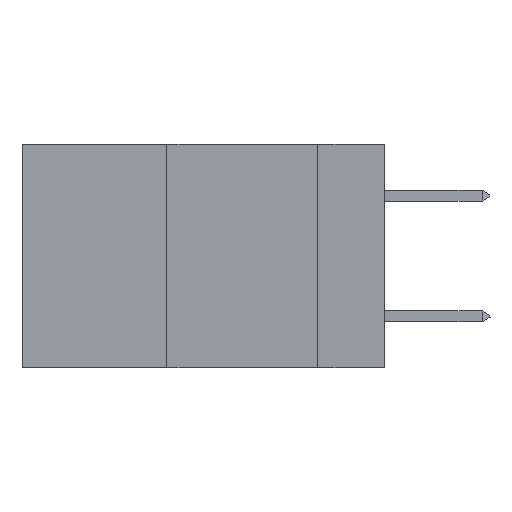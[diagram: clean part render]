
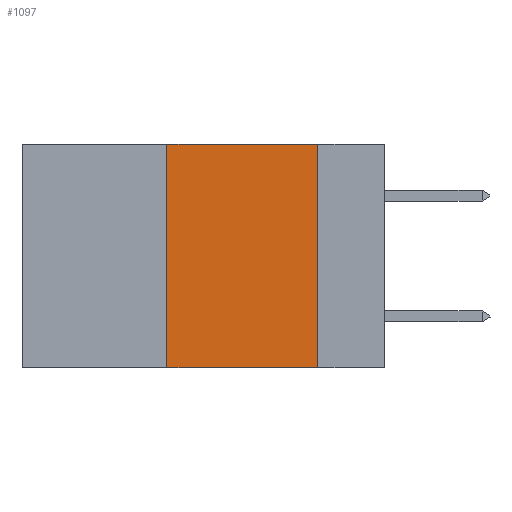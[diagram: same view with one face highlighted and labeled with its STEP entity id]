
A CAD part, left-side view. The second image highlights one B-rep face of the part: STEP entity #1097.
In plain terms, the highlighted planar face has unit normal (-1, 0, 0).
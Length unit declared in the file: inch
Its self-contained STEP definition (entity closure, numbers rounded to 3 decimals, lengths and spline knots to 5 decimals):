
#472 = CARTESIAN_POINT ( 'NONE',  ( 0., 0.36, 0. ) ) ;
#550 = VECTOR ( 'NONE', #9578, 39.37008 ) ;
#721 = VECTOR ( 'NONE', #6037, 39.37008 ) ;
#830 = EDGE_LOOP ( 'NONE', ( #2233, #8775, #4856, #7892 ) ) ;
#1097 = ADVANCED_FACE ( 'NONE', ( #7365 ), #3379, .F. ) ;
#1171 = EDGE_CURVE ( 'NONE', #7683, #2452, #3147, .T. ) ;
#1399 = CARTESIAN_POINT ( 'NONE',  ( 0., 0.36, -0.37 ) ) ;
#2233 = ORIENTED_EDGE ( 'NONE', *, *, #5070, .F. ) ;
#2452 = VERTEX_POINT ( 'NONE', #7179 ) ;
#3147 = LINE ( 'NONE', #7239, #550 ) ;
#3379 = PLANE ( 'NONE',  #5464 ) ;
#3863 = VECTOR ( 'NONE', #4103, 39.37008 ) ;
#4103 = DIRECTION ( 'NONE',  ( 0., -1., 0. ) ) ;
#4136 = VECTOR ( 'NONE', #4860, 39.37008 ) ;
#4198 = DIRECTION ( 'NONE',  ( 1., 0., 0. ) ) ;
#4224 = VERTEX_POINT ( 'NONE', #472 ) ;
#4382 = LINE ( 'NONE', #9440, #4136 ) ;
#4623 = VERTEX_POINT ( 'NONE', #6936 ) ;
#4636 = CARTESIAN_POINT ( 'NONE',  ( 0., 0.36, 0. ) ) ;
#4856 = ORIENTED_EDGE ( 'NONE', *, *, #9575, .F. ) ;
#4860 = DIRECTION ( 'NONE',  ( 0., 0., -1. ) ) ;
#5070 = EDGE_CURVE ( 'NONE', #4623, #2452, #4382, .T. ) ;
#5464 = AXIS2_PLACEMENT_3D ( 'NONE', #8773, #4198, #5795 ) ;
#5795 = DIRECTION ( 'NONE',  ( 0., 0., -1. ) ) ;
#6037 = DIRECTION ( 'NONE',  ( 0., 0., 1. ) ) ;
#6936 = CARTESIAN_POINT ( 'NONE',  ( 0., 0.11, 0. ) ) ;
#7095 = EDGE_CURVE ( 'NONE', #4224, #4623, #7511, .T. ) ;
#7179 = CARTESIAN_POINT ( 'NONE',  ( 0., 0.11, -0.37 ) ) ;
#7239 = CARTESIAN_POINT ( 'NONE',  ( 0., 0.6, -0.37 ) ) ;
#7365 = FACE_OUTER_BOUND ( 'NONE', #830, .T. ) ;
#7511 = LINE ( 'NONE', #9426, #3863 ) ;
#7683 = VERTEX_POINT ( 'NONE', #1399 ) ;
#7892 = ORIENTED_EDGE ( 'NONE', *, *, #1171, .T. ) ;
#8027 = LINE ( 'NONE', #4636, #721 ) ;
#8773 = CARTESIAN_POINT ( 'NONE',  ( 0., 0.6, 0. ) ) ;
#8775 = ORIENTED_EDGE ( 'NONE', *, *, #7095, .F. ) ;
#9426 = CARTESIAN_POINT ( 'NONE',  ( 0., 0.6, 0. ) ) ;
#9440 = CARTESIAN_POINT ( 'NONE',  ( 0., 0.11, 0. ) ) ;
#9575 = EDGE_CURVE ( 'NONE', #7683, #4224, #8027, .T. ) ;
#9578 = DIRECTION ( 'NONE',  ( 0., -1., 0. ) ) ;
